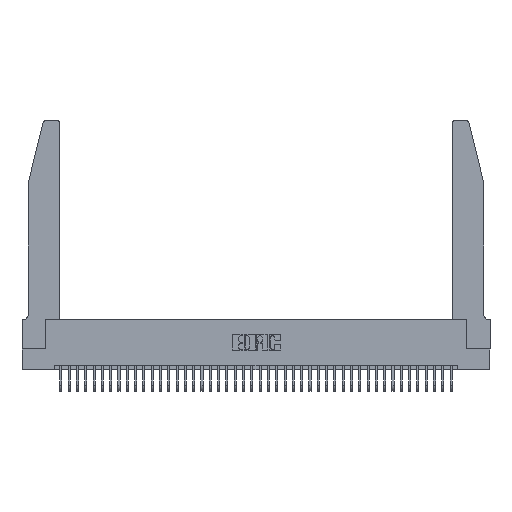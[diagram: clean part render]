
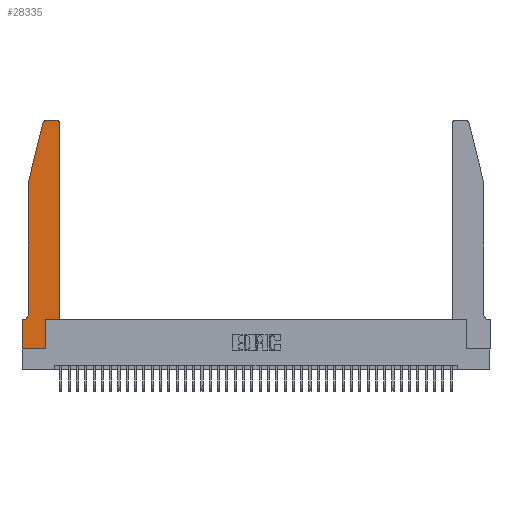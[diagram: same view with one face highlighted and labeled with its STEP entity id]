
A CAD part, top view. The second image highlights one B-rep face of the part: STEP entity #28335.
In plain terms, the highlighted planar face has unit normal (0, 0, 1).
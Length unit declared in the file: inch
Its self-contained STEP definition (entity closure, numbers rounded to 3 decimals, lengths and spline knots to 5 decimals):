
#1060 = CARTESIAN_POINT ( 'NONE',  ( 0.2865, 0.35, 0.37 ) ) ;
#1229 = DIRECTION ( 'NONE',  ( 1., 0., 0. ) ) ;
#1686 = ORIENTED_EDGE ( 'NONE', *, *, #26466, .T. ) ;
#2054 = ORIENTED_EDGE ( 'NONE', *, *, #36043, .T. ) ;
#2241 = CARTESIAN_POINT ( 'NONE',  ( 0.4505, 2.72, 0.37 ) ) ;
#2701 = ORIENTED_EDGE ( 'NONE', *, *, #39986, .T. ) ;
#3469 = CIRCLE ( 'NONE', #27936, 0.07 ) ;
#3851 = CARTESIAN_POINT ( 'NONE',  ( 0.25487, 2.72718, 0.37 ) ) ;
#3866 = AXIS2_PLACEMENT_3D ( 'NONE', #18111, #41451, #21452 ) ;
#4237 = VERTEX_POINT ( 'NONE', #33687 ) ;
#4951 = VERTEX_POINT ( 'NONE', #30420 ) ;
#5125 = CARTESIAN_POINT ( 'NONE',  ( 0.0755, 2., 0.37 ) ) ;
#5183 = EDGE_CURVE ( 'NONE', #28721, #29488, #30668, .T. ) ;
#5307 = CARTESIAN_POINT ( 'NONE',  ( 0.0755, 2., 0.37 ) ) ;
#5879 = CARTESIAN_POINT ( 'NONE',  ( 0., 0., 0.37 ) ) ;
#6432 = VERTEX_POINT ( 'NONE', #1060 ) ;
#6756 = EDGE_CURVE ( 'NONE', #4237, #39653, #32085, .T. ) ;
#7437 = VERTEX_POINT ( 'NONE', #33178 ) ;
#7662 = CARTESIAN_POINT ( 'NONE',  ( 0., 0.35, 0.37 ) ) ;
#7828 = CARTESIAN_POINT ( 'NONE',  ( 0.4505, 0.35, 0.37 ) ) ;
#8500 = DIRECTION ( 'NONE',  ( 0., -1., 0. ) ) ;
#8680 = DIRECTION ( 'NONE',  ( -0.239, -0.971, 0. ) ) ;
#8766 = CIRCLE ( 'NONE', #18018, 0.03 ) ;
#9270 = DIRECTION ( 'NONE',  ( 0., -1., 0. ) ) ;
#9808 = ORIENTED_EDGE ( 'NONE', *, *, #31923, .T. ) ;
#9961 = CARTESIAN_POINT ( 'NONE',  ( 0.0055, 0.42, 0.37 ) ) ;
#10295 = VERTEX_POINT ( 'NONE', #2241 ) ;
#10510 = ORIENTED_EDGE ( 'NONE', *, *, #6756, .T. ) ;
#10661 = CARTESIAN_POINT ( 'NONE',  ( 0.0055, 0.35, 0.37 ) ) ;
#10939 = VECTOR ( 'NONE', #8680, 39.37008 ) ;
#11278 = CARTESIAN_POINT ( 'NONE',  ( 0.284, 2.72, 0.37 ) ) ;
#12755 = CARTESIAN_POINT ( 'NONE',  ( 0.2865, 0., 0.37 ) ) ;
#13312 = DIRECTION ( 'NONE',  ( -1., 0., 0. ) ) ;
#13968 = VECTOR ( 'NONE', #34792, 39.37008 ) ;
#14347 = VECTOR ( 'NONE', #42840, 39.37008 ) ;
#14440 = FACE_OUTER_BOUND ( 'NONE', #20848, .T. ) ;
#14627 = DIRECTION ( 'NONE',  ( 1., 0., 0. ) ) ;
#14803 = LINE ( 'NONE', #7828, #41414 ) ;
#14806 = CARTESIAN_POINT ( 'NONE',  ( 0.0755, 0.35, 0.37 ) ) ;
#15364 = CARTESIAN_POINT ( 'NONE',  ( 0.4505, 0.35, 0.37 ) ) ;
#15718 = ORIENTED_EDGE ( 'NONE', *, *, #40805, .T. ) ;
#16011 = CARTESIAN_POINT ( 'NONE',  ( 0., 0., 0.37 ) ) ;
#16130 = VECTOR ( 'NONE', #8500, 39.37008 ) ;
#17899 = AXIS2_PLACEMENT_3D ( 'NONE', #19504, #42850, #22872 ) ;
#17942 = CARTESIAN_POINT ( 'NONE',  ( 0.2605, 2.75, 0.37 ) ) ;
#18018 = AXIS2_PLACEMENT_3D ( 'NONE', #11278, #34604, #14627 ) ;
#18111 = CARTESIAN_POINT ( 'NONE',  ( 0., 0.35, 0.37 ) ) ;
#18765 = LINE ( 'NONE', #17942, #36668 ) ;
#19193 = EDGE_CURVE ( 'NONE', #6432, #7437, #14803, .T. ) ;
#19504 = CARTESIAN_POINT ( 'NONE',  ( 0.4205, 2.72, 0.37 ) ) ;
#20848 = EDGE_LOOP ( 'NONE', ( #9808, #37710, #15718, #1686, #38639, #37521, #22756, #10510, #2701, #39785, #2054, #42367 ) ) ;
#21452 = DIRECTION ( 'NONE',  ( 1., 0., 0. ) ) ;
#21792 = VERTEX_POINT ( 'NONE', #3851 ) ;
#22173 = LINE ( 'NONE', #23836, #38901 ) ;
#22756 = ORIENTED_EDGE ( 'NONE', *, *, #32832, .T. ) ;
#22872 = DIRECTION ( 'NONE',  ( 1., 0., 0. ) ) ;
#23836 = CARTESIAN_POINT ( 'NONE',  ( 0.2865, 0.35, 0.37 ) ) ;
#26466 = EDGE_CURVE ( 'NONE', #37393, #4951, #33878, .T. ) ;
#27154 = DIRECTION ( 'NONE',  ( 0., 1., 0. ) ) ;
#27936 = AXIS2_PLACEMENT_3D ( 'NONE', #9961, #33295, #13312 ) ;
#28115 = DIRECTION ( 'NONE',  ( -1., 0., 0. ) ) ;
#28139 = VECTOR ( 'NONE', #9270, 39.37008 ) ;
#28335 = ADVANCED_FACE ( 'NONE', ( #14440 ), #31401, .T. ) ;
#28597 = DIRECTION ( 'NONE',  ( 0., 1., 0. ) ) ;
#28633 = LINE ( 'NONE', #5307, #10939 ) ;
#28721 = VERTEX_POINT ( 'NONE', #10661 ) ;
#29037 = CARTESIAN_POINT ( 'NONE',  ( 0.284, 2.75, 0.37 ) ) ;
#29173 = EDGE_CURVE ( 'NONE', #10295, #33887, #35245, .T. ) ;
#29194 = LINE ( 'NONE', #5879, #28139 ) ;
#29488 = VERTEX_POINT ( 'NONE', #7662 ) ;
#30420 = CARTESIAN_POINT ( 'NONE',  ( 0.0755, 0.42, 0.37 ) ) ;
#30668 = LINE ( 'NONE', #14806, #13968 ) ;
#31401 = PLANE ( 'NONE',  #3866 ) ;
#31923 = EDGE_CURVE ( 'NONE', #33887, #41614, #18765, .T. ) ;
#32085 = LINE ( 'NONE', #16011, #14347 ) ;
#32832 = EDGE_CURVE ( 'NONE', #29488, #4237, #29194, .T. ) ;
#33178 = CARTESIAN_POINT ( 'NONE',  ( 0.4505, 0.35, 0.37 ) ) ;
#33202 = LINE ( 'NONE', #15364, #41020 ) ;
#33295 = DIRECTION ( 'NONE',  ( 0., 0., -1. ) ) ;
#33687 = CARTESIAN_POINT ( 'NONE',  ( 0., 0., 0.37 ) ) ;
#33878 = LINE ( 'NONE', #5125, #16130 ) ;
#33887 = VERTEX_POINT ( 'NONE', #34228 ) ;
#34228 = CARTESIAN_POINT ( 'NONE',  ( 0.4205, 2.75, 0.37 ) ) ;
#34604 = DIRECTION ( 'NONE',  ( 0., 0., 1. ) ) ;
#34625 = EDGE_CURVE ( 'NONE', #41614, #21792, #8766, .T. ) ;
#34792 = DIRECTION ( 'NONE',  ( -1., 0., 0. ) ) ;
#35245 = CIRCLE ( 'NONE', #17899, 0.03 ) ;
#36043 = EDGE_CURVE ( 'NONE', #7437, #10295, #33202, .T. ) ;
#36668 = VECTOR ( 'NONE', #28115, 39.37008 ) ;
#37393 = VERTEX_POINT ( 'NONE', #42692 ) ;
#37521 = ORIENTED_EDGE ( 'NONE', *, *, #5183, .T. ) ;
#37710 = ORIENTED_EDGE ( 'NONE', *, *, #34625, .T. ) ;
#38639 = ORIENTED_EDGE ( 'NONE', *, *, #41974, .T. ) ;
#38901 = VECTOR ( 'NONE', #27154, 39.37008 ) ;
#39653 = VERTEX_POINT ( 'NONE', #12755 ) ;
#39785 = ORIENTED_EDGE ( 'NONE', *, *, #19193, .T. ) ;
#39986 = EDGE_CURVE ( 'NONE', #39653, #6432, #22173, .T. ) ;
#40805 = EDGE_CURVE ( 'NONE', #21792, #37393, #28633, .T. ) ;
#41020 = VECTOR ( 'NONE', #28597, 39.37008 ) ;
#41414 = VECTOR ( 'NONE', #1229, 39.37008 ) ;
#41451 = DIRECTION ( 'NONE',  ( 0., 0., 1. ) ) ;
#41614 = VERTEX_POINT ( 'NONE', #29037 ) ;
#41974 = EDGE_CURVE ( 'NONE', #4951, #28721, #3469, .T. ) ;
#42367 = ORIENTED_EDGE ( 'NONE', *, *, #29173, .T. ) ;
#42692 = CARTESIAN_POINT ( 'NONE',  ( 0.0755, 2., 0.37 ) ) ;
#42840 = DIRECTION ( 'NONE',  ( 1., 0., 0. ) ) ;
#42850 = DIRECTION ( 'NONE',  ( 0., 0., 1. ) ) ;
